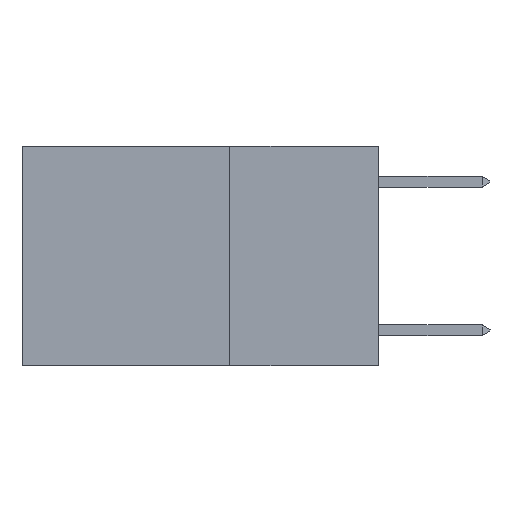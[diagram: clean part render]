
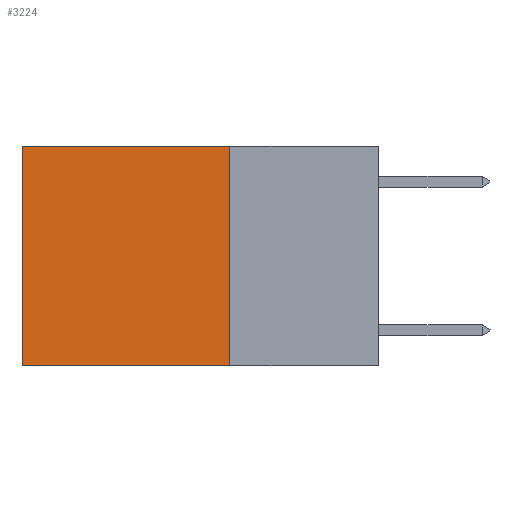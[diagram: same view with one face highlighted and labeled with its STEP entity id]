
A CAD part, left-side view. The second image highlights one B-rep face of the part: STEP entity #3224.
In plain terms, the highlighted planar face has unit normal (-1, 0, 0).
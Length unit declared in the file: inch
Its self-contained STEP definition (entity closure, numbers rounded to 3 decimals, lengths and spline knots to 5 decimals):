
#128 = VECTOR ( 'NONE', #10178, 39.37008 ) ;
#721 = LINE ( 'NONE', #15985, #8171 ) ;
#1055 = LINE ( 'NONE', #2397, #4602 ) ;
#1068 = VERTEX_POINT ( 'NONE', #13343 ) ;
#1584 = ORIENTED_EDGE ( 'NONE', *, *, #5846, .T. ) ;
#2039 = ORIENTED_EDGE ( 'NONE', *, *, #5391, .F. ) ;
#2397 = CARTESIAN_POINT ( 'NONE',  ( 0.2625, 0.6, 0. ) ) ;
#3224 = ADVANCED_FACE ( 'NONE', ( #10346 ), #4594, .F. ) ;
#3316 = EDGE_CURVE ( 'NONE', #15389, #10474, #721, .T. ) ;
#3929 = CARTESIAN_POINT ( 'NONE',  ( 0.2625, 0.6, 0. ) ) ;
#3981 = CARTESIAN_POINT ( 'NONE',  ( 0.2625, 0.25, 0. ) ) ;
#4300 = ORIENTED_EDGE ( 'NONE', *, *, #3316, .F. ) ;
#4494 = ORIENTED_EDGE ( 'NONE', *, *, #7161, .T. ) ;
#4594 = PLANE ( 'NONE',  #14482 ) ;
#4602 = VECTOR ( 'NONE', #8290, 39.37008 ) ;
#5391 = EDGE_CURVE ( 'NONE', #10474, #1068, #11766, .T. ) ;
#5846 = EDGE_CURVE ( 'NONE', #11305, #1068, #1055, .T. ) ;
#6052 = CARTESIAN_POINT ( 'NONE',  ( 0.2625, 0.25, 0. ) ) ;
#6250 = LINE ( 'NONE', #3981, #9644 ) ;
#6850 = CARTESIAN_POINT ( 'NONE',  ( 0.2625, 0.25, -0.37 ) ) ;
#7161 = EDGE_CURVE ( 'NONE', #15389, #11305, #6250, .T. ) ;
#7542 = DIRECTION ( 'NONE',  ( 1., 0., 0. ) ) ;
#7730 = DIRECTION ( 'NONE',  ( 0., 0., -1. ) ) ;
#8171 = VECTOR ( 'NONE', #7730, 39.37008 ) ;
#8290 = DIRECTION ( 'NONE',  ( 0., 0., -1. ) ) ;
#8781 = CARTESIAN_POINT ( 'NONE',  ( 0.2625, 0.25, -0.37 ) ) ;
#9469 = CARTESIAN_POINT ( 'NONE',  ( 0.2625, 0.25, 0. ) ) ;
#9644 = VECTOR ( 'NONE', #15287, 39.37008 ) ;
#10174 = EDGE_LOOP ( 'NONE', ( #1584, #2039, #4300, #4494 ) ) ;
#10178 = DIRECTION ( 'NONE',  ( 0., 1., 0. ) ) ;
#10346 = FACE_OUTER_BOUND ( 'NONE', #10174, .T. ) ;
#10474 = VERTEX_POINT ( 'NONE', #6850 ) ;
#11305 = VERTEX_POINT ( 'NONE', #3929 ) ;
#11766 = LINE ( 'NONE', #8781, #128 ) ;
#13343 = CARTESIAN_POINT ( 'NONE',  ( 0.2625, 0.6, -0.37 ) ) ;
#14482 = AXIS2_PLACEMENT_3D ( 'NONE', #6052, #7542, #17095 ) ;
#15287 = DIRECTION ( 'NONE',  ( 0., 1., 0. ) ) ;
#15389 = VERTEX_POINT ( 'NONE', #9469 ) ;
#15985 = CARTESIAN_POINT ( 'NONE',  ( 0.2625, 0.25, 0. ) ) ;
#17095 = DIRECTION ( 'NONE',  ( 0., 0., -1. ) ) ;
